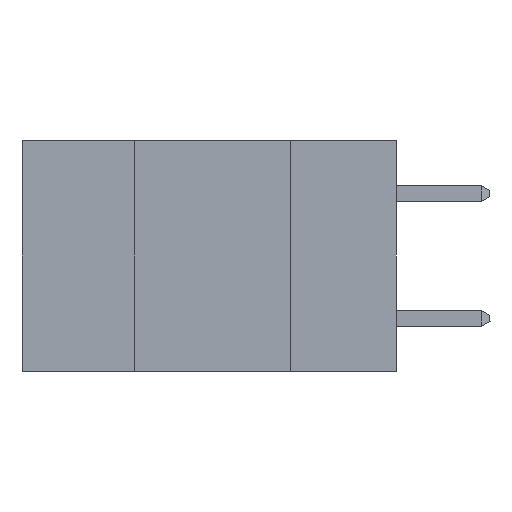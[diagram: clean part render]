
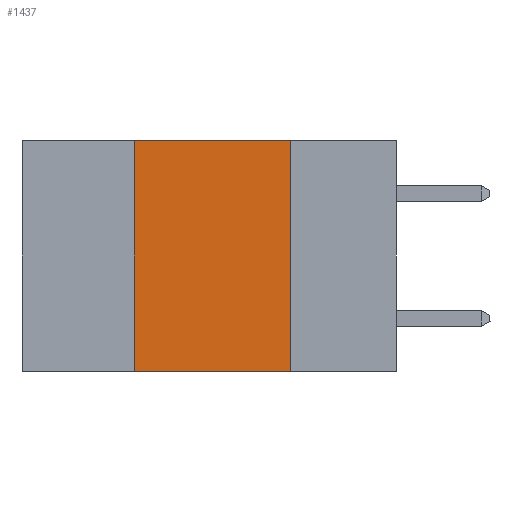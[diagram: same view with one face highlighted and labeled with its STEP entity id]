
A CAD part, left-side view. The second image highlights one B-rep face of the part: STEP entity #1437.
In plain terms, the highlighted planar face has unit normal (-1, 0, 0).
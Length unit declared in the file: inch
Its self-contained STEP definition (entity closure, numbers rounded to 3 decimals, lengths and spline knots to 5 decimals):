
#233 = FACE_OUTER_BOUND ( 'NONE', #7177, .T. ) ;
#463 = CARTESIAN_POINT ( 'NONE',  ( 0., 0.6, 0. ) ) ;
#932 = EDGE_CURVE ( 'NONE', #8227, #3088, #4536, .T. ) ;
#1437 = ADVANCED_FACE ( 'NONE', ( #233 ), #9138, .F. ) ;
#1476 = CARTESIAN_POINT ( 'NONE',  ( 0., 0.42, -0.37 ) ) ;
#1600 = CARTESIAN_POINT ( 'NONE',  ( 0., 0.6, -0.37 ) ) ;
#1743 = LINE ( 'NONE', #463, #7803 ) ;
#1988 = VERTEX_POINT ( 'NONE', #8882 ) ;
#2074 = DIRECTION ( 'NONE',  ( 0., -1., 0. ) ) ;
#2133 = EDGE_CURVE ( 'NONE', #8227, #7595, #4393, .T. ) ;
#2283 = LINE ( 'NONE', #4767, #7976 ) ;
#2873 = DIRECTION ( 'NONE',  ( 1., 0., 0. ) ) ;
#3007 = CARTESIAN_POINT ( 'NONE',  ( 0., 0.17, -0.37 ) ) ;
#3088 = VERTEX_POINT ( 'NONE', #3179 ) ;
#3093 = DIRECTION ( 'NONE',  ( 0., 0., 1. ) ) ;
#3179 = CARTESIAN_POINT ( 'NONE',  ( 0., 0.42, 0. ) ) ;
#3274 = DIRECTION ( 'NONE',  ( 0., -1., 0. ) ) ;
#3674 = DIRECTION ( 'NONE',  ( 0., 0., -1. ) ) ;
#4222 = EDGE_CURVE ( 'NONE', #1988, #7595, #2283, .T. ) ;
#4393 = LINE ( 'NONE', #1600, #5251 ) ;
#4536 = LINE ( 'NONE', #1476, #6558 ) ;
#4589 = AXIS2_PLACEMENT_3D ( 'NONE', #7588, #2873, #3674 ) ;
#4767 = CARTESIAN_POINT ( 'NONE',  ( 0., 0.17, -0.37 ) ) ;
#5251 = VECTOR ( 'NONE', #3274, 39.37008 ) ;
#6558 = VECTOR ( 'NONE', #3093, 39.37008 ) ;
#6563 = EDGE_CURVE ( 'NONE', #3088, #1988, #1743, .T. ) ;
#7157 = ORIENTED_EDGE ( 'NONE', *, *, #4222, .F. ) ;
#7177 = EDGE_LOOP ( 'NONE', ( #7157, #8153, #7598, #8548 ) ) ;
#7588 = CARTESIAN_POINT ( 'NONE',  ( 0., 0.6, 0. ) ) ;
#7595 = VERTEX_POINT ( 'NONE', #3007 ) ;
#7598 = ORIENTED_EDGE ( 'NONE', *, *, #932, .F. ) ;
#7678 = CARTESIAN_POINT ( 'NONE',  ( 0., 0.42, -0.37 ) ) ;
#7803 = VECTOR ( 'NONE', #2074, 39.37008 ) ;
#7976 = VECTOR ( 'NONE', #8711, 39.37008 ) ;
#8153 = ORIENTED_EDGE ( 'NONE', *, *, #6563, .F. ) ;
#8227 = VERTEX_POINT ( 'NONE', #7678 ) ;
#8548 = ORIENTED_EDGE ( 'NONE', *, *, #2133, .T. ) ;
#8711 = DIRECTION ( 'NONE',  ( 0., 0., -1. ) ) ;
#8882 = CARTESIAN_POINT ( 'NONE',  ( 0., 0.17, 0. ) ) ;
#9138 = PLANE ( 'NONE',  #4589 ) ;
